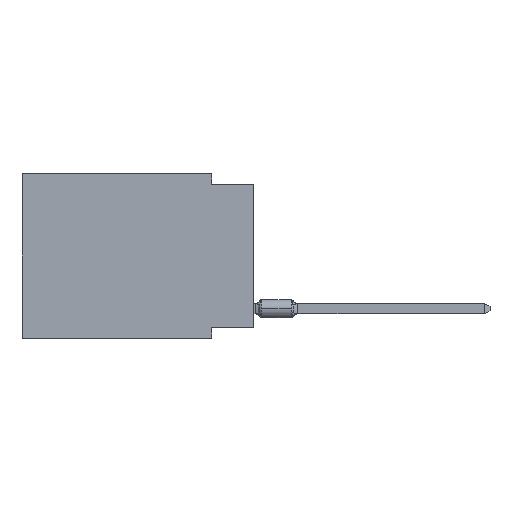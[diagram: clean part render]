
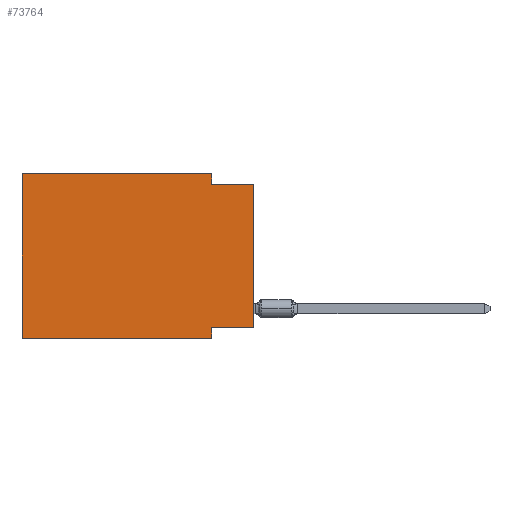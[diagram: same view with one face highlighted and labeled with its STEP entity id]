
A CAD part, left-side view. The second image highlights one B-rep face of the part: STEP entity #73764.
In plain terms, the highlighted planar face has unit normal (-1, 0, 0).
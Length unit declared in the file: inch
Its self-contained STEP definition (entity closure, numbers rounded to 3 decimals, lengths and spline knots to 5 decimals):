
#187 = VECTOR ( 'NONE', #65945, 39.37008 ) ;
#3638 = DIRECTION ( 'NONE',  ( 1., 0., 0. ) ) ;
#4025 = DIRECTION ( 'NONE',  ( 0., 0., -1. ) ) ;
#5115 = CARTESIAN_POINT ( 'NONE',  ( 0., 0., -0.365 ) ) ;
#8394 = ORIENTED_EDGE ( 'NONE', *, *, #35777, .F. ) ;
#13560 = AXIS2_PLACEMENT_3D ( 'NONE', #40194, #3638, #4025 ) ;
#14235 = DIRECTION ( 'NONE',  ( 0., -1., 0. ) ) ;
#15116 = FACE_OUTER_BOUND ( 'NONE', #66126, .T. ) ;
#15215 = VECTOR ( 'NONE', #71020, 39.37008 ) ;
#15665 = VECTOR ( 'NONE', #19070, 39.37008 ) ;
#18489 = EDGE_CURVE ( 'NONE', #71856, #41694, #61844, .T. ) ;
#19070 = DIRECTION ( 'NONE',  ( 0., 0., 1. ) ) ;
#21331 = DIRECTION ( 'NONE',  ( 0., 0., 1. ) ) ;
#23124 = VERTEX_POINT ( 'NONE', #67771 ) ;
#23336 = DIRECTION ( 'NONE',  ( 0., -1., 0. ) ) ;
#23584 = CARTESIAN_POINT ( 'NONE',  ( 0., 0., -0.365 ) ) ;
#26476 = VECTOR ( 'NONE', #30971, 39.37008 ) ;
#26667 = CARTESIAN_POINT ( 'NONE',  ( 0., 0.55, 0. ) ) ;
#27665 = CARTESIAN_POINT ( 'NONE',  ( 0., 0.55, -0.39 ) ) ;
#27840 = CARTESIAN_POINT ( 'NONE',  ( 0., 0.1, -0.365 ) ) ;
#30971 = DIRECTION ( 'NONE',  ( 0., -1., 0. ) ) ;
#32740 = LINE ( 'NONE', #57817, #66246 ) ;
#34599 = EDGE_CURVE ( 'NONE', #71856, #78012, #81125, .T. ) ;
#35777 = EDGE_CURVE ( 'NONE', #62413, #23124, #64460, .T. ) ;
#36318 = CARTESIAN_POINT ( 'NONE',  ( 0., 0.55, -0.39 ) ) ;
#36876 = ORIENTED_EDGE ( 'NONE', *, *, #58610, .F. ) ;
#38202 = CARTESIAN_POINT ( 'NONE',  ( 0., 0., -0.025 ) ) ;
#38492 = VECTOR ( 'NONE', #23336, 39.37008 ) ;
#38547 = VECTOR ( 'NONE', #21331, 39.37008 ) ;
#38710 = ORIENTED_EDGE ( 'NONE', *, *, #43052, .F. ) ;
#40194 = CARTESIAN_POINT ( 'NONE',  ( 0., 0.55, 0. ) ) ;
#40532 = EDGE_CURVE ( 'NONE', #78012, #56608, #61406, .T. ) ;
#40599 = PLANE ( 'NONE',  #13560 ) ;
#41312 = VECTOR ( 'NONE', #41682, 39.37008 ) ;
#41650 = ORIENTED_EDGE ( 'NONE', *, *, #18489, .T. ) ;
#41682 = DIRECTION ( 'NONE',  ( 0., 1., 0. ) ) ;
#41694 = VERTEX_POINT ( 'NONE', #38202 ) ;
#42334 = ORIENTED_EDGE ( 'NONE', *, *, #34599, .F. ) ;
#43052 = EDGE_CURVE ( 'NONE', #71081, #50317, #78458, .T. ) ;
#43440 = CARTESIAN_POINT ( 'NONE',  ( 0., 0.55, 0. ) ) ;
#49871 = ORIENTED_EDGE ( 'NONE', *, *, #50485, .F. ) ;
#50317 = VERTEX_POINT ( 'NONE', #43440 ) ;
#50485 = EDGE_CURVE ( 'NONE', #50317, #62413, #32740, .T. ) ;
#51600 = CARTESIAN_POINT ( 'NONE',  ( 0., 0.1, 0. ) ) ;
#52116 = CARTESIAN_POINT ( 'NONE',  ( 0., 0.1, 0. ) ) ;
#53941 = CARTESIAN_POINT ( 'NONE',  ( 0., 0.1, -0.39 ) ) ;
#54574 = LINE ( 'NONE', #59140, #38492 ) ;
#55234 = LINE ( 'NONE', #36318, #26476 ) ;
#55735 = ORIENTED_EDGE ( 'NONE', *, *, #40532, .F. ) ;
#56608 = VERTEX_POINT ( 'NONE', #53941 ) ;
#57817 = CARTESIAN_POINT ( 'NONE',  ( 0., 0.55, 0. ) ) ;
#58610 = EDGE_CURVE ( 'NONE', #23124, #41694, #54574, .T. ) ;
#59140 = CARTESIAN_POINT ( 'NONE',  ( 0., 0., -0.025 ) ) ;
#59450 = ORIENTED_EDGE ( 'NONE', *, *, #71891, .T. ) ;
#60587 = CARTESIAN_POINT ( 'NONE',  ( 0., 0.1, -0.39 ) ) ;
#61406 = LINE ( 'NONE', #60587, #187 ) ;
#61844 = LINE ( 'NONE', #74168, #15665 ) ;
#62413 = VERTEX_POINT ( 'NONE', #51600 ) ;
#64460 = LINE ( 'NONE', #52116, #15215 ) ;
#65945 = DIRECTION ( 'NONE',  ( 0., 0., -1. ) ) ;
#66126 = EDGE_LOOP ( 'NONE', ( #41650, #36876, #8394, #49871, #38710, #59450, #55735, #42334 ) ) ;
#66246 = VECTOR ( 'NONE', #14235, 39.37008 ) ;
#67771 = CARTESIAN_POINT ( 'NONE',  ( 0., 0.1, -0.025 ) ) ;
#71020 = DIRECTION ( 'NONE',  ( 0., 0., -1. ) ) ;
#71081 = VERTEX_POINT ( 'NONE', #27665 ) ;
#71856 = VERTEX_POINT ( 'NONE', #23584 ) ;
#71891 = EDGE_CURVE ( 'NONE', #71081, #56608, #55234, .T. ) ;
#73764 = ADVANCED_FACE ( 'NONE', ( #15116 ), #40599, .F. ) ;
#74168 = CARTESIAN_POINT ( 'NONE',  ( 0., 0., 0. ) ) ;
#78012 = VERTEX_POINT ( 'NONE', #27840 ) ;
#78458 = LINE ( 'NONE', #26667, #38547 ) ;
#81125 = LINE ( 'NONE', #5115, #41312 ) ;
